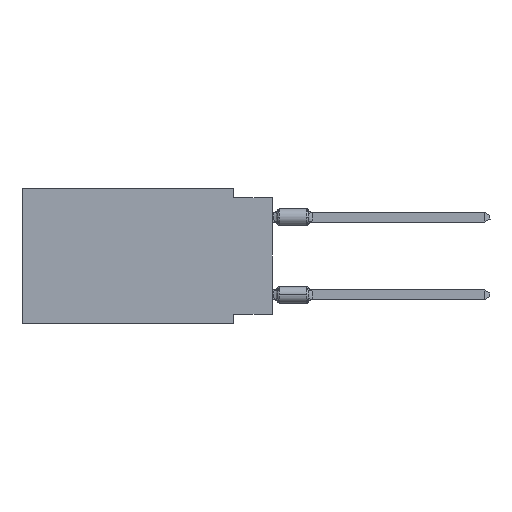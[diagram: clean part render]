
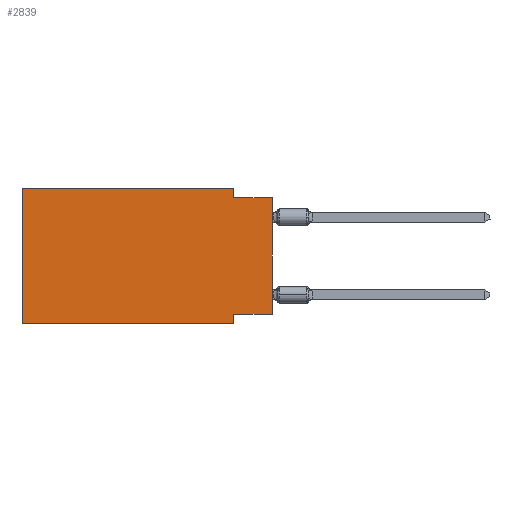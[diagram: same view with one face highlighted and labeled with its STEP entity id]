
A CAD part, left-side view. The second image highlights one B-rep face of the part: STEP entity #2839.
In plain terms, the highlighted planar face has unit normal (-1, 0, 0).
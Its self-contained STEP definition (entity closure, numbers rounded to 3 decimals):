
#393 = FACE_OUTER_BOUND ( 'NONE', #1214, .T. ) ;
#747 = LINE ( 'NONE', #18403, #45399 ) ;
#1214 = EDGE_LOOP ( 'NONE', ( #37445, #8165, #1777, #2440, #25823, #32969, #38363, #3014 ) ) ;
#1544 = PLANE ( 'NONE',  #19237 ) ;
#1777 = ORIENTED_EDGE ( 'NONE', *, *, #29499, .F. ) ;
#1852 = EDGE_CURVE ( 'NONE', #45351, #44086, #21399, .T. ) ;
#2080 = CARTESIAN_POINT ( 'NONE',  ( 0., 2.54, 0. ) ) ;
#2440 = ORIENTED_EDGE ( 'NONE', *, *, #13600, .F. ) ;
#2839 = ADVANCED_FACE ( 'NONE', ( #393 ), #1544, .F. ) ;
#3014 = ORIENTED_EDGE ( 'NONE', *, *, #19708, .F. ) ;
#3083 = CARTESIAN_POINT ( 'NONE',  ( 0., 16.383, -8.89 ) ) ;
#3233 = VERTEX_POINT ( 'NONE', #18011 ) ;
#4248 = CARTESIAN_POINT ( 'NONE',  ( 0., 2.54, -0.635 ) ) ;
#4341 = EDGE_CURVE ( 'NONE', #34594, #27349, #32867, .T. ) ;
#4704 = DIRECTION ( 'NONE',  ( 0., 0., 1. ) ) ;
#5085 = DIRECTION ( 'NONE',  ( 0., 0., -1. ) ) ;
#5177 = CARTESIAN_POINT ( 'NONE',  ( 0., 0., -0.635 ) ) ;
#8165 = ORIENTED_EDGE ( 'NONE', *, *, #4341, .F. ) ;
#8973 = VERTEX_POINT ( 'NONE', #2080 ) ;
#10128 = CARTESIAN_POINT ( 'NONE',  ( 0., 0., -8.255 ) ) ;
#12352 = LINE ( 'NONE', #37447, #16273 ) ;
#13600 = EDGE_CURVE ( 'NONE', #24448, #8973, #41643, .T. ) ;
#14976 = CARTESIAN_POINT ( 'NONE',  ( 0., 0., -8.255 ) ) ;
#15988 = EDGE_CURVE ( 'NONE', #3233, #44086, #26381, .T. ) ;
#16273 = VECTOR ( 'NONE', #4704, 1000. ) ;
#18011 = CARTESIAN_POINT ( 'NONE',  ( 0., 2.54, -8.255 ) ) ;
#18146 = VECTOR ( 'NONE', #29145, 1000. ) ;
#18403 = CARTESIAN_POINT ( 'NONE',  ( 0., 2.54, 0. ) ) ;
#19103 = VECTOR ( 'NONE', #38852, 1000. ) ;
#19237 = AXIS2_PLACEMENT_3D ( 'NONE', #40808, #33619, #23353 ) ;
#19708 = EDGE_CURVE ( 'NONE', #22511, #3233, #29831, .T. ) ;
#21233 = LINE ( 'NONE', #28459, #44595 ) ;
#21399 = LINE ( 'NONE', #3083, #31001 ) ;
#22511 = VERTEX_POINT ( 'NONE', #10128 ) ;
#23353 = DIRECTION ( 'NONE',  ( 0., 0., -1. ) ) ;
#24448 = VERTEX_POINT ( 'NONE', #42369 ) ;
#24946 = DIRECTION ( 'NONE',  ( 0., 0., 1. ) ) ;
#25823 = ORIENTED_EDGE ( 'NONE', *, *, #43077, .F. ) ;
#26334 = DIRECTION ( 'NONE',  ( 0., -1., 0. ) ) ;
#26381 = LINE ( 'NONE', #30778, #43665 ) ;
#27349 = VERTEX_POINT ( 'NONE', #41875 ) ;
#28408 = DIRECTION ( 'NONE',  ( 0., -1., 0. ) ) ;
#28459 = CARTESIAN_POINT ( 'NONE',  ( 0., 16.383, 0. ) ) ;
#29145 = DIRECTION ( 'NONE',  ( 0., 1., 0. ) ) ;
#29499 = EDGE_CURVE ( 'NONE', #8973, #34594, #747, .T. ) ;
#29831 = LINE ( 'NONE', #14976, #18146 ) ;
#30778 = CARTESIAN_POINT ( 'NONE',  ( 0., 2.54, -8.89 ) ) ;
#31001 = VECTOR ( 'NONE', #28408, 1000. ) ;
#31836 = EDGE_CURVE ( 'NONE', #22511, #27349, #12352, .T. ) ;
#31850 = CARTESIAN_POINT ( 'NONE',  ( 0., 16.383, 0. ) ) ;
#32867 = LINE ( 'NONE', #5177, #39384 ) ;
#32969 = ORIENTED_EDGE ( 'NONE', *, *, #1852, .T. ) ;
#33619 = DIRECTION ( 'NONE',  ( 1., 0., 0. ) ) ;
#34594 = VERTEX_POINT ( 'NONE', #4248 ) ;
#37074 = DIRECTION ( 'NONE',  ( 0., 0., -1. ) ) ;
#37445 = ORIENTED_EDGE ( 'NONE', *, *, #31836, .T. ) ;
#37447 = CARTESIAN_POINT ( 'NONE',  ( 0., 0., 0. ) ) ;
#38363 = ORIENTED_EDGE ( 'NONE', *, *, #15988, .F. ) ;
#38852 = DIRECTION ( 'NONE',  ( 0., -1., 0. ) ) ;
#39384 = VECTOR ( 'NONE', #26334, 1000. ) ;
#40808 = CARTESIAN_POINT ( 'NONE',  ( 0., 16.383, 0. ) ) ;
#41643 = LINE ( 'NONE', #31850, #19103 ) ;
#41875 = CARTESIAN_POINT ( 'NONE',  ( 0., 0., -0.635 ) ) ;
#42001 = CARTESIAN_POINT ( 'NONE',  ( 0., 16.383, -8.89 ) ) ;
#42212 = CARTESIAN_POINT ( 'NONE',  ( 0., 2.54, -8.89 ) ) ;
#42369 = CARTESIAN_POINT ( 'NONE',  ( 0., 16.383, 0. ) ) ;
#43077 = EDGE_CURVE ( 'NONE', #45351, #24448, #21233, .T. ) ;
#43665 = VECTOR ( 'NONE', #37074, 1000. ) ;
#44086 = VERTEX_POINT ( 'NONE', #42212 ) ;
#44595 = VECTOR ( 'NONE', #24946, 1000. ) ;
#45351 = VERTEX_POINT ( 'NONE', #42001 ) ;
#45399 = VECTOR ( 'NONE', #5085, 1000. ) ;
